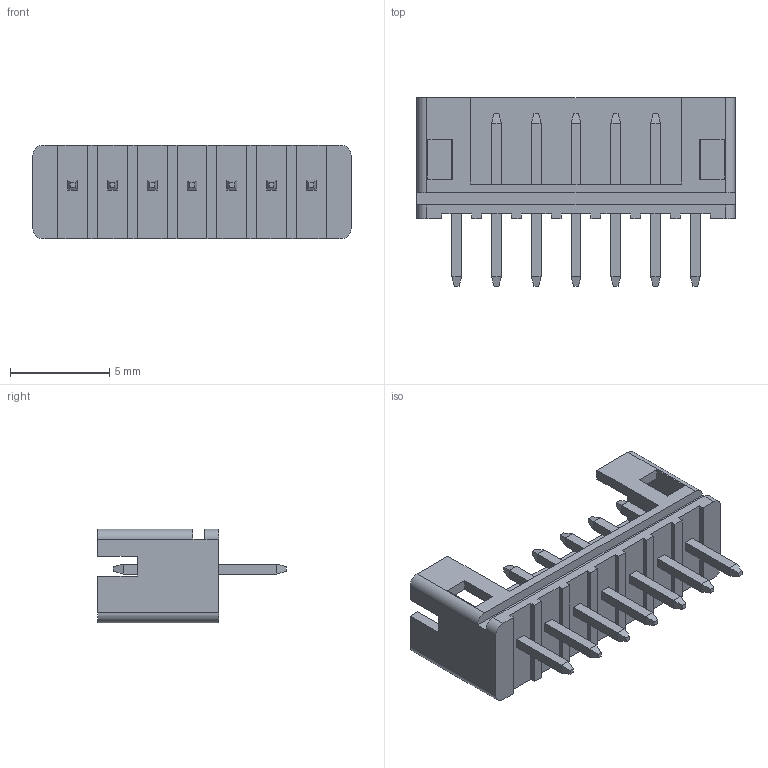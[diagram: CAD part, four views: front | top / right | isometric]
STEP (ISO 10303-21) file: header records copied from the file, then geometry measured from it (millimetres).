
FILE_DESCRIPTION (( 'STEP AP203' ), '1' );
FILE_NAME ('140-507-415-101.STEP', '2020-09-25T11:17:00', ( '' ), ( '' ), 'SwSTEP 2.0', 'SolidWorks 2020', '' );
FILE_SCHEMA (( 'CONFIG_CONTROL_DESIGN' ));
Length unit declared in the file: millimetre
Products named in the file (3): V LI Contact_Str; V LI Housing_507; 140-507-415-101
Assembly tree (8 placements, depth 2):
  140-507-415-101
    V LI Housing_507
    V LI Contact_Str  x7
Bounding box: 16 x 9.5 x 4.7 mm (x, y, z)
Volume: 175.8 mm3; surface area: 644.6 mm2
Topology: 8 solids, 8 shells, 194 faces, 480 edges, 300 vertices
Faces by surface type: plane 188, cylinder 6
Entity records: 4025 total; most frequent: CARTESIAN_POINT 637, ORIENTED_EDGE 624, DIRECTION 566, EDGE_CURVE 312, LINE 300, VECTOR 300, VERTEX_POINT 204, AXIS2_PLACEMENT_3D 133
